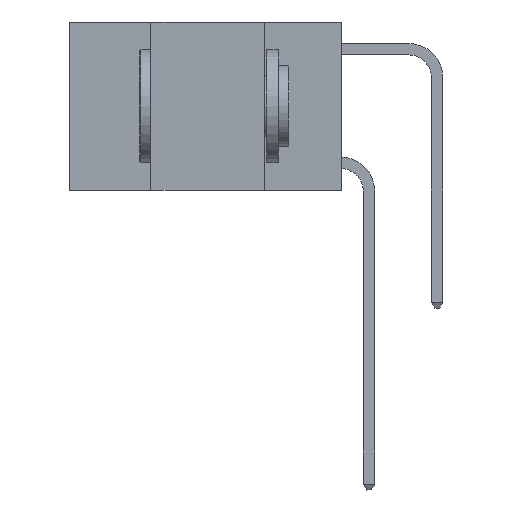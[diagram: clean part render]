
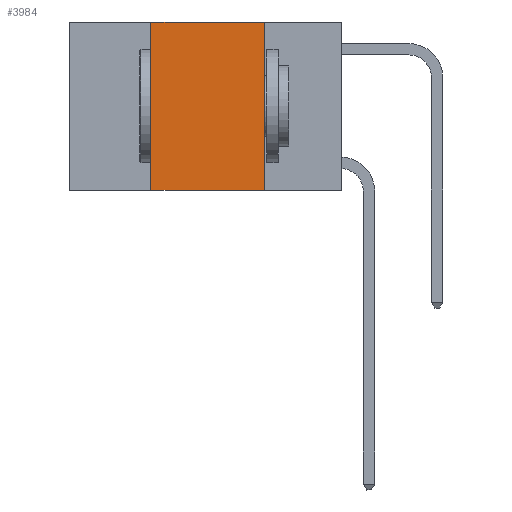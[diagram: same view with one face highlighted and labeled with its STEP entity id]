
A CAD part, left-side view. The second image highlights one B-rep face of the part: STEP entity #3984.
In plain terms, the highlighted planar face has unit normal (-1, 0, 0).
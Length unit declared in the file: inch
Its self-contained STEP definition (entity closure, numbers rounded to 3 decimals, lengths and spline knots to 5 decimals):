
#1764 = CARTESIAN_POINT ( 'NONE',  ( 0., 0.6, -0.37 ) ) ;
#1802 = CARTESIAN_POINT ( 'NONE',  ( 0., 0.17, -0.37 ) ) ;
#2789 = DIRECTION ( 'NONE',  ( 0., -1., 0. ) ) ;
#2795 = VERTEX_POINT ( 'NONE', #29717 ) ;
#2947 = LINE ( 'NONE', #28105, #8396 ) ;
#3984 = ADVANCED_FACE ( 'NONE', ( #18000 ), #22801, .F. ) ;
#4228 = CARTESIAN_POINT ( 'NONE',  ( 0., 0.6, 0. ) ) ;
#4893 = DIRECTION ( 'NONE',  ( 0., 0., 1. ) ) ;
#5748 = LINE ( 'NONE', #12040, #11178 ) ;
#8396 = VECTOR ( 'NONE', #4893, 39.37008 ) ;
#8541 = VERTEX_POINT ( 'NONE', #1802 ) ;
#8585 = VERTEX_POINT ( 'NONE', #15907 ) ;
#8881 = DIRECTION ( 'NONE',  ( 1., 0., 0. ) ) ;
#9907 = ORIENTED_EDGE ( 'NONE', *, *, #20868, .T. ) ;
#10472 = ORIENTED_EDGE ( 'NONE', *, *, #12556, .F. ) ;
#10686 = VERTEX_POINT ( 'NONE', #18735 ) ;
#11178 = VECTOR ( 'NONE', #2789, 39.37008 ) ;
#11560 = AXIS2_PLACEMENT_3D ( 'NONE', #4228, #8881, #25135 ) ;
#11775 = LINE ( 'NONE', #29853, #17226 ) ;
#12040 = CARTESIAN_POINT ( 'NONE',  ( 0., 0.6, 0. ) ) ;
#12556 = EDGE_CURVE ( 'NONE', #2795, #8541, #11775, .T. ) ;
#13661 = DIRECTION ( 'NONE',  ( 0., 0., -1. ) ) ;
#14651 = ORIENTED_EDGE ( 'NONE', *, *, #23883, .F. ) ;
#15764 = DIRECTION ( 'NONE',  ( 0., -1., 0. ) ) ;
#15907 = CARTESIAN_POINT ( 'NONE',  ( 0., 0.42, -0.37 ) ) ;
#16918 = EDGE_CURVE ( 'NONE', #8585, #10686, #2947, .T. ) ;
#17226 = VECTOR ( 'NONE', #13661, 39.37008 ) ;
#18000 = FACE_OUTER_BOUND ( 'NONE', #21287, .T. ) ;
#18735 = CARTESIAN_POINT ( 'NONE',  ( 0., 0.42, 0. ) ) ;
#20560 = LINE ( 'NONE', #1764, #25998 ) ;
#20868 = EDGE_CURVE ( 'NONE', #8585, #8541, #20560, .T. ) ;
#21287 = EDGE_LOOP ( 'NONE', ( #10472, #14651, #22981, #9907 ) ) ;
#22801 = PLANE ( 'NONE',  #11560 ) ;
#22981 = ORIENTED_EDGE ( 'NONE', *, *, #16918, .F. ) ;
#23883 = EDGE_CURVE ( 'NONE', #10686, #2795, #5748, .T. ) ;
#25135 = DIRECTION ( 'NONE',  ( 0., 0., -1. ) ) ;
#25998 = VECTOR ( 'NONE', #15764, 39.37008 ) ;
#28105 = CARTESIAN_POINT ( 'NONE',  ( 0., 0.42, 0. ) ) ;
#29717 = CARTESIAN_POINT ( 'NONE',  ( 0., 0.17, 0. ) ) ;
#29853 = CARTESIAN_POINT ( 'NONE',  ( 0., 0.17, 0. ) ) ;
